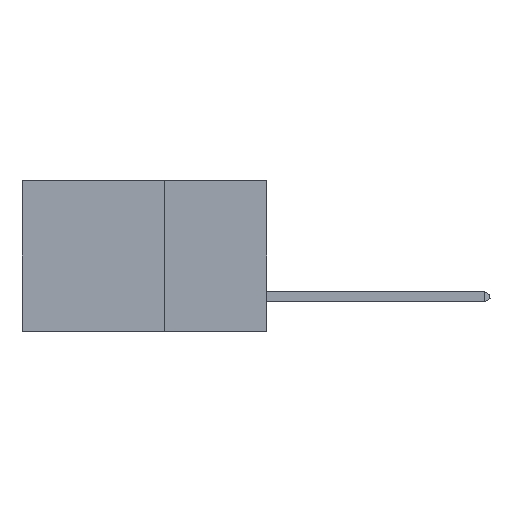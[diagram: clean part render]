
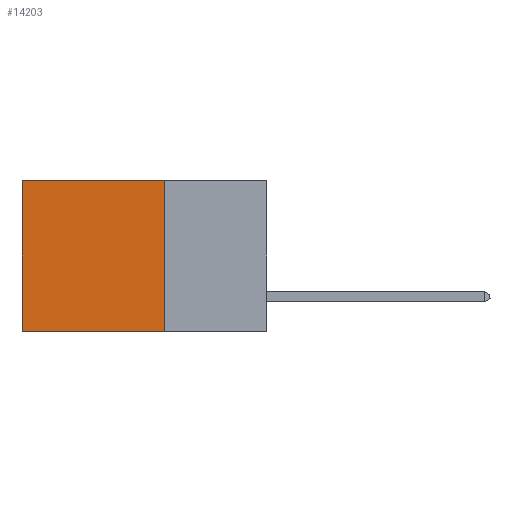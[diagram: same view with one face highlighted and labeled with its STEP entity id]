
A CAD part, left-side view. The second image highlights one B-rep face of the part: STEP entity #14203.
In plain terms, the highlighted planar face has unit normal (-1, 0, 0).
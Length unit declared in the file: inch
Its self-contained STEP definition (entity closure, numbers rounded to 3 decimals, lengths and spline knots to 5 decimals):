
#66 = FACE_OUTER_BOUND ( 'NONE', #11881, .T. ) ;
#1832 = CARTESIAN_POINT ( 'NONE',  ( 0.2875, 0.6, 0. ) ) ;
#2795 = VERTEX_POINT ( 'NONE', #1832 ) ;
#2908 = CARTESIAN_POINT ( 'NONE',  ( 0.2875, 0.25, 0. ) ) ;
#3411 = VECTOR ( 'NONE', #11116, 39.37008 ) ;
#3549 = DIRECTION ( 'NONE',  ( 1., 0., 0. ) ) ;
#3635 = ORIENTED_EDGE ( 'NONE', *, *, #11016, .F. ) ;
#3910 = DIRECTION ( 'NONE',  ( 0., 1., 0. ) ) ;
#4320 = EDGE_CURVE ( 'NONE', #11582, #7783, #15213, .T. ) ;
#4337 = DIRECTION ( 'NONE',  ( 0., 0., -1. ) ) ;
#4830 = DIRECTION ( 'NONE',  ( 0., 0., -1. ) ) ;
#4930 = DIRECTION ( 'NONE',  ( 0., 0., -1. ) ) ;
#5835 = LINE ( 'NONE', #2908, #13701 ) ;
#6036 = AXIS2_PLACEMENT_3D ( 'NONE', #6774, #3549, #4830 ) ;
#6774 = CARTESIAN_POINT ( 'NONE',  ( 0.2875, 0.25, 0. ) ) ;
#7026 = CARTESIAN_POINT ( 'NONE',  ( 0.2875, 0.6, -0.37 ) ) ;
#7483 = CARTESIAN_POINT ( 'NONE',  ( 0.2875, 0.25, 0. ) ) ;
#7783 = VERTEX_POINT ( 'NONE', #7026 ) ;
#7950 = ORIENTED_EDGE ( 'NONE', *, *, #10685, .T. ) ;
#8835 = ORIENTED_EDGE ( 'NONE', *, *, #14560, .T. ) ;
#10018 = CARTESIAN_POINT ( 'NONE',  ( 0.2875, 0.25, -0.37 ) ) ;
#10327 = LINE ( 'NONE', #11006, #11107 ) ;
#10632 = ORIENTED_EDGE ( 'NONE', *, *, #4320, .F. ) ;
#10685 = EDGE_CURVE ( 'NONE', #2795, #7783, #10327, .T. ) ;
#10936 = VERTEX_POINT ( 'NONE', #7483 ) ;
#11006 = CARTESIAN_POINT ( 'NONE',  ( 0.2875, 0.6, 0. ) ) ;
#11016 = EDGE_CURVE ( 'NONE', #10936, #11582, #5835, .T. ) ;
#11107 = VECTOR ( 'NONE', #4930, 39.37008 ) ;
#11116 = DIRECTION ( 'NONE',  ( 0., 1., 0. ) ) ;
#11307 = LINE ( 'NONE', #11318, #14844 ) ;
#11318 = CARTESIAN_POINT ( 'NONE',  ( 0.2875, 0.25, 0. ) ) ;
#11582 = VERTEX_POINT ( 'NONE', #10018 ) ;
#11881 = EDGE_LOOP ( 'NONE', ( #7950, #10632, #3635, #8835 ) ) ;
#11887 = PLANE ( 'NONE',  #6036 ) ;
#12250 = CARTESIAN_POINT ( 'NONE',  ( 0.2875, 0.25, -0.37 ) ) ;
#13701 = VECTOR ( 'NONE', #4337, 39.37008 ) ;
#14203 = ADVANCED_FACE ( 'NONE', ( #66 ), #11887, .F. ) ;
#14560 = EDGE_CURVE ( 'NONE', #10936, #2795, #11307, .T. ) ;
#14844 = VECTOR ( 'NONE', #3910, 39.37008 ) ;
#15213 = LINE ( 'NONE', #12250, #3411 ) ;
